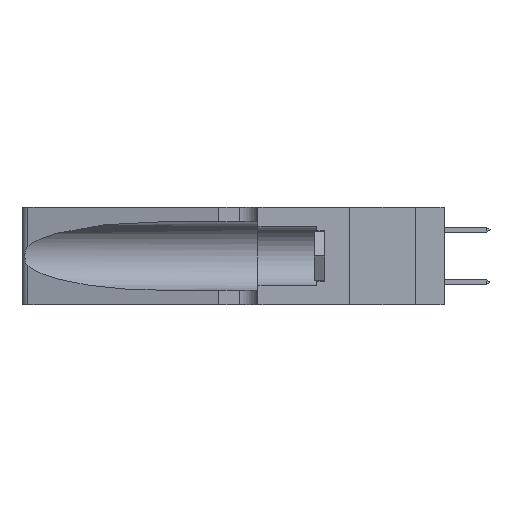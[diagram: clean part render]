
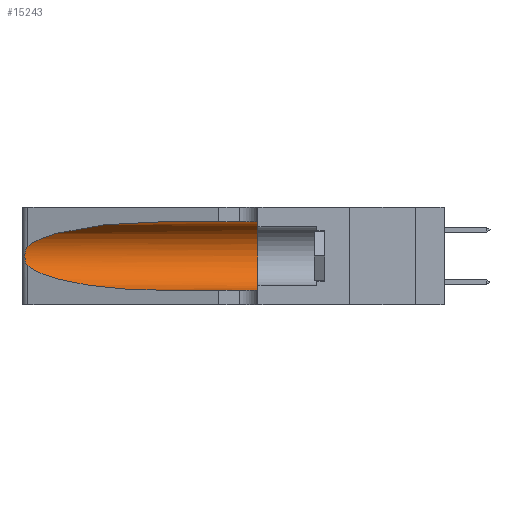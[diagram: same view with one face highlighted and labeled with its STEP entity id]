
A CAD part, left-side view. The second image highlights one B-rep face of the part: STEP entity #15243.
In plain terms, the highlighted cylindrical face has radius 3.308 mm (diameter 6.617 mm), a partial arc.
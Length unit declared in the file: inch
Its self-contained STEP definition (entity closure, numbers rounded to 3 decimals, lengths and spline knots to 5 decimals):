
#168 = CARTESIAN_POINT ( 'NONE',  ( 0.1305, 0.72297, 0.05475 ) ) ;
#1380 = VERTEX_POINT ( 'NONE', #2762 ) ;
#1427 = ORIENTED_EDGE ( 'NONE', *, *, #8331, .T. ) ;
#1556 = CARTESIAN_POINT ( 'NONE',  ( 0.25639, 1.23184, 0.21858 ) ) ;
#2762 = CARTESIAN_POINT ( 'NONE',  ( 0.1305, 0.35, 0.31525 ) ) ;
#2787 = EDGE_CURVE ( 'NONE', #8462, #14023, #11717, .T. ) ;
#2967 = B_SPLINE_CURVE_WITH_KNOTS ( 'NONE', 3,
 ( #7820, #16795, #1556, #12340, #3143, #13827, #4757, #15331, #6351, #16858, #7879, #18331, #9417, #17349 ),
 .UNSPECIFIED., .F., .F.,
 ( 4, 2, 2, 2, 2, 2, 4 ),
 ( 0., 0.00027, 0.00053, 0.00107, 0.0016, 0.00187, 0.00214 ),
 .UNSPECIFIED. ) ;
#3143 = CARTESIAN_POINT ( 'NONE',  ( 0.25854, 1.2359, 0.20912 ) ) ;
#3227 = EDGE_CURVE ( 'NONE', #1380, #14023, #4051, .T. ) ;
#3777 = ORIENTED_EDGE ( 'NONE', *, *, #2787, .T. ) ;
#3800 = LINE ( 'NONE', #7488, #19365 ) ;
#4051 = CIRCLE ( 'NONE', #11308, 0.13025 ) ;
#4240 = CARTESIAN_POINT ( 'NONE',  ( 0.1305, 1.61858, 0.185 ) ) ;
#4440 = DIRECTION ( 'NONE',  ( 0., -1., 0. ) ) ;
#4455 = FACE_OUTER_BOUND ( 'NONE', #4560, .T. ) ;
#4560 = EDGE_LOOP ( 'NONE', ( #1427, #10698, #5471, #3777, #19381, #17085 ) ) ;
#4757 = CARTESIAN_POINT ( 'NONE',  ( 0.26075, 1.23896, 0.19203 ) ) ;
#5471 = ORIENTED_EDGE ( 'NONE', *, *, #18020, .T. ) ;
#5820 = VERTEX_POINT ( 'NONE', #15939 ) ;
#5930 = CARTESIAN_POINT ( 'NONE',  ( 0.25487, 1.22718, 0.22369 ) ) ;
#5982 = DIRECTION ( 'NONE',  ( 0., -1., 0. ) ) ;
#6014 = DIRECTION ( 'NONE',  ( 0., 0., -1. ) ) ;
#6351 = CARTESIAN_POINT ( 'NONE',  ( 0.26017, 1.23833, 0.17102 ) ) ;
#6567 = CARTESIAN_POINT ( 'NONE',  ( 0.25487, 1.22718, 0.14631 ) ) ;
#7475 = CARTESIAN_POINT ( 'NONE',  ( 0.18966, 0.96281, 0.31525 ) ) ;
#7488 = CARTESIAN_POINT ( 'NONE',  ( 0.1305, 1.61858, 0.31525 ) ) ;
#7820 = CARTESIAN_POINT ( 'NONE',  ( 0.25487, 1.22718, 0.22369 ) ) ;
#7879 = CARTESIAN_POINT ( 'NONE',  ( 0.25789, 1.23486, 0.15765 ) ) ;
#8223 = DIRECTION ( 'NONE',  ( 0., 1., 0. ) ) ;
#8250 = DIRECTION ( 'NONE',  ( 0., 0., 1. ) ) ;
#8331 = EDGE_CURVE ( 'NONE', #16946, #16622, #9292, .T. ) ;
#8462 = VERTEX_POINT ( 'NONE', #9324 ) ;
#9205 = CARTESIAN_POINT ( 'NONE',  ( 0.1305, 0.35, 0.185 ) ) ;
#9292 =( BOUNDED_CURVE ( )  B_SPLINE_CURVE ( 3, ( #19410, #7475, #16447, #10515 ),
 .UNSPECIFIED., .F., .F. ) 
 B_SPLINE_CURVE_WITH_KNOTS ( ( 4, 4 ),
 ( 1.5708, 2.84003 ),
 .UNSPECIFIED. ) 
 CURVE ( )  GEOMETRIC_REPRESENTATION_ITEM ( )  RATIONAL_B_SPLINE_CURVE ( ( 1., 0.87, 0.87, 1. ) ) 
 REPRESENTATION_ITEM ( '' )  );
#9324 = CARTESIAN_POINT ( 'NONE',  ( 0.1305, 0.72297, 0.05475 ) ) ;
#9417 = CARTESIAN_POINT ( 'NONE',  ( 0.25555, 1.22993, 0.14849 ) ) ;
#9610 = CARTESIAN_POINT ( 'NONE',  ( 0.18966, 0.96281, 0.05475 ) ) ;
#10515 = CARTESIAN_POINT ( 'NONE',  ( 0.25487, 1.22718, 0.22369 ) ) ;
#10698 = ORIENTED_EDGE ( 'NONE', *, *, #13634, .T. ) ;
#10976 = CARTESIAN_POINT ( 'NONE',  ( 0.1305, 1.61858, 0.05475 ) ) ;
#11149 = CARTESIAN_POINT ( 'NONE',  ( 0.1305, 0.72297, 0.31525 ) ) ;
#11308 = AXIS2_PLACEMENT_3D ( 'NONE', #9205, #8223, #8250 ) ;
#11717 = LINE ( 'NONE', #10976, #19605 ) ;
#12186 = AXIS2_PLACEMENT_3D ( 'NONE', #4240, #4440, #6014 ) ;
#12340 = CARTESIAN_POINT ( 'NONE',  ( 0.25787, 1.23484, 0.2124 ) ) ;
#12911 = CYLINDRICAL_SURFACE ( 'NONE', #12186, 0.13025 ) ;
#13634 = EDGE_CURVE ( 'NONE', #16622, #5820, #2967, .T. ) ;
#13827 = CARTESIAN_POINT ( 'NONE',  ( 0.26018, 1.23835, 0.19895 ) ) ;
#14023 = VERTEX_POINT ( 'NONE', #19224 ) ;
#15243 = ADVANCED_FACE ( 'NONE', ( #4455 ), #12911, .F. ) ;
#15331 = CARTESIAN_POINT ( 'NONE',  ( 0.26075, 1.23896, 0.178 ) ) ;
#15588 =( BOUNDED_CURVE ( )  B_SPLINE_CURVE ( 3, ( #6567, #18526, #9610, #168 ),
 .UNSPECIFIED., .F., .F. ) 
 B_SPLINE_CURVE_WITH_KNOTS ( ( 4, 4 ),
 ( 3.44316, 4.71239 ),
 .UNSPECIFIED. ) 
 CURVE ( )  GEOMETRIC_REPRESENTATION_ITEM ( )  RATIONAL_B_SPLINE_CURVE ( ( 1., 0.87, 0.87, 1. ) ) 
 REPRESENTATION_ITEM ( '' )  );
#15939 = CARTESIAN_POINT ( 'NONE',  ( 0.25487, 1.22718, 0.14631 ) ) ;
#16447 = CARTESIAN_POINT ( 'NONE',  ( 0.2373, 1.15595, 0.28018 ) ) ;
#16516 = DIRECTION ( 'NONE',  ( 0., -1., 0. ) ) ;
#16622 = VERTEX_POINT ( 'NONE', #5930 ) ;
#16649 = EDGE_CURVE ( 'NONE', #16946, #1380, #3800, .T. ) ;
#16795 = CARTESIAN_POINT ( 'NONE',  ( 0.25555, 1.22994, 0.2215 ) ) ;
#16858 = CARTESIAN_POINT ( 'NONE',  ( 0.25856, 1.23593, 0.16098 ) ) ;
#16946 = VERTEX_POINT ( 'NONE', #11149 ) ;
#17085 = ORIENTED_EDGE ( 'NONE', *, *, #16649, .F. ) ;
#17349 = CARTESIAN_POINT ( 'NONE',  ( 0.25487, 1.22718, 0.14631 ) ) ;
#18020 = EDGE_CURVE ( 'NONE', #5820, #8462, #15588, .T. ) ;
#18331 = CARTESIAN_POINT ( 'NONE',  ( 0.25639, 1.23186, 0.15144 ) ) ;
#18526 = CARTESIAN_POINT ( 'NONE',  ( 0.2373, 1.15595, 0.08982 ) ) ;
#19224 = CARTESIAN_POINT ( 'NONE',  ( 0.1305, 0.35, 0.05475 ) ) ;
#19365 = VECTOR ( 'NONE', #16516, 39.37008 ) ;
#19381 = ORIENTED_EDGE ( 'NONE', *, *, #3227, .F. ) ;
#19410 = CARTESIAN_POINT ( 'NONE',  ( 0.1305, 0.72297, 0.31525 ) ) ;
#19605 = VECTOR ( 'NONE', #5982, 39.37008 ) ;
